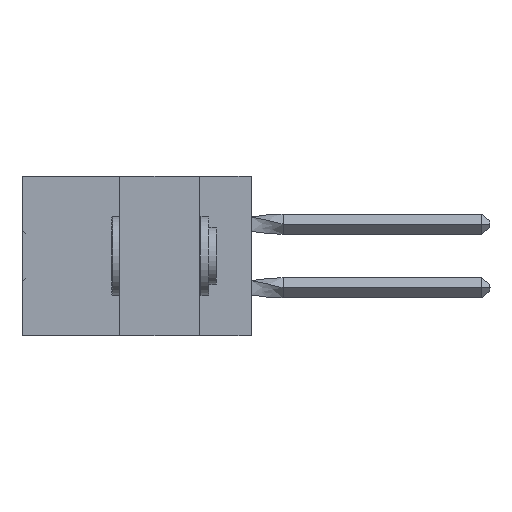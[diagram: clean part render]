
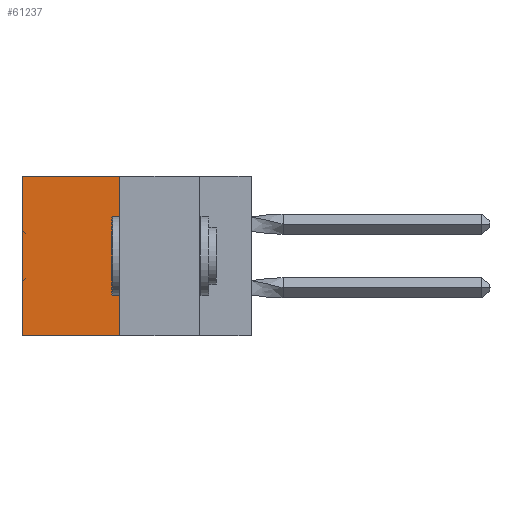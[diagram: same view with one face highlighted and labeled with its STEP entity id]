
A CAD part, left-side view. The second image highlights one B-rep face of the part: STEP entity #61237.
In plain terms, the highlighted planar face has unit normal (-1, 0, 0).
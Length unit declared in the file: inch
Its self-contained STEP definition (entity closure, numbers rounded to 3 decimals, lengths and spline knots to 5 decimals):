
#546 = DIRECTION ( 'NONE',  ( 0., 0., -1. ) ) ;
#972 = DIRECTION ( 'NONE',  ( 1., 0., 0. ) ) ;
#2047 = LINE ( 'NONE', #14438, #13166 ) ;
#2955 = VERTEX_POINT ( 'NONE', #42833 ) ;
#2965 = EDGE_CURVE ( 'NONE', #12762, #23542, #2047, .T. ) ;
#6923 = LINE ( 'NONE', #40313, #39556 ) ;
#12762 = VERTEX_POINT ( 'NONE', #25641 ) ;
#13166 = VECTOR ( 'NONE', #28747, 39.37008 ) ;
#14257 = CARTESIAN_POINT ( 'NONE',  ( 0.305, 0.413, -0.5 ) ) ;
#14438 = CARTESIAN_POINT ( 'NONE',  ( 0.305, 0.413, 0. ) ) ;
#14887 = ORIENTED_EDGE ( 'NONE', *, *, #21448, .T. ) ;
#16724 = DIRECTION ( 'NONE',  ( 0., 1., 0. ) ) ;
#16850 = ORIENTED_EDGE ( 'NONE', *, *, #57726, .F. ) ;
#16949 = ORIENTED_EDGE ( 'NONE', *, *, #2965, .T. ) ;
#18459 = CARTESIAN_POINT ( 'NONE',  ( 0.305, 0.413, -0.5 ) ) ;
#21448 = EDGE_CURVE ( 'NONE', #23542, #2955, #41095, .T. ) ;
#22176 = EDGE_CURVE ( 'NONE', #12762, #38822, #29227, .T. ) ;
#23542 = VERTEX_POINT ( 'NONE', #50065 ) ;
#23857 = DIRECTION ( 'NONE',  ( 0., 0., -1. ) ) ;
#25641 = CARTESIAN_POINT ( 'NONE',  ( 0.305, 0.413, 0. ) ) ;
#28347 = DIRECTION ( 'NONE',  ( 0., 0., -1. ) ) ;
#28747 = DIRECTION ( 'NONE',  ( 0., 1., 0. ) ) ;
#29227 = LINE ( 'NONE', #14257, #38092 ) ;
#36047 = FACE_OUTER_BOUND ( 'NONE', #58927, .T. ) ;
#38092 = VECTOR ( 'NONE', #28347, 39.37008 ) ;
#38446 = PLANE ( 'NONE',  #44227 ) ;
#38822 = VERTEX_POINT ( 'NONE', #18459 ) ;
#38938 = VECTOR ( 'NONE', #23857, 39.37008 ) ;
#39556 = VECTOR ( 'NONE', #16724, 39.37008 ) ;
#40313 = CARTESIAN_POINT ( 'NONE',  ( 0.305, 0.413, -0.5 ) ) ;
#41095 = LINE ( 'NONE', #42683, #38938 ) ;
#42683 = CARTESIAN_POINT ( 'NONE',  ( 0.305, 0.72, -0.5 ) ) ;
#42833 = CARTESIAN_POINT ( 'NONE',  ( 0.305, 0.72, -0.5 ) ) ;
#43018 = CARTESIAN_POINT ( 'NONE',  ( 0.305, 0.413, -0.5 ) ) ;
#44227 = AXIS2_PLACEMENT_3D ( 'NONE', #43018, #972, #546 ) ;
#50065 = CARTESIAN_POINT ( 'NONE',  ( 0.305, 0.72, 0. ) ) ;
#51054 = ORIENTED_EDGE ( 'NONE', *, *, #22176, .F. ) ;
#57726 = EDGE_CURVE ( 'NONE', #38822, #2955, #6923, .T. ) ;
#58927 = EDGE_LOOP ( 'NONE', ( #14887, #16850, #51054, #16949 ) ) ;
#61237 = ADVANCED_FACE ( 'NONE', ( #36047 ), #38446, .F. ) ;
